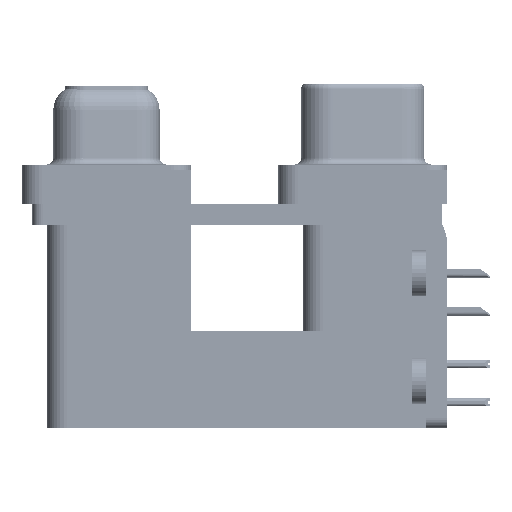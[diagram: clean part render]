
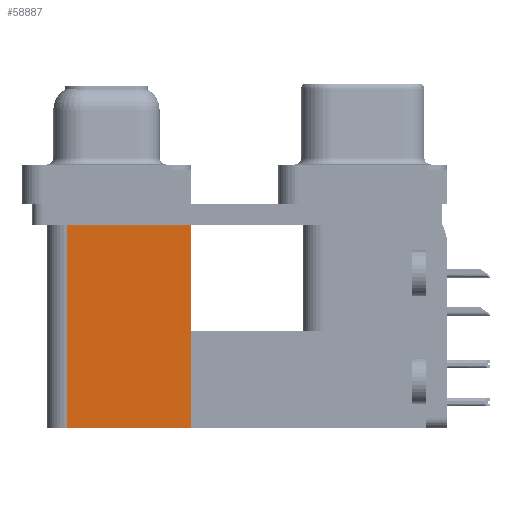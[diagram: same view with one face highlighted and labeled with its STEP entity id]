
A CAD part, left-side view. The second image highlights one B-rep face of the part: STEP entity #58887.
In plain terms, the highlighted planar face has unit normal (-1, 0, 0).
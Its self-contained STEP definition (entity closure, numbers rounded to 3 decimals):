
#113 = CARTESIAN_POINT ( 'NONE',  ( 3.79, 12.775, -19.2 ) ) ;
#594 = VECTOR ( 'NONE', #69800, 1000. ) ;
#6363 = VERTEX_POINT ( 'NONE', #7071 ) ;
#7071 = CARTESIAN_POINT ( 'NONE',  ( 3.79, 21.975, -2.5 ) ) ;
#8855 = DIRECTION ( 'NONE',  ( 0., 1., 0. ) ) ;
#9341 = ORIENTED_EDGE ( 'NONE', *, *, #26535, .T. ) ;
#10146 = EDGE_CURVE ( 'NONE', #29169, #64016, #26181, .T. ) ;
#14301 = VECTOR ( 'NONE', #15058, 1000. ) ;
#15058 = DIRECTION ( 'NONE',  ( 0., 1., 0. ) ) ;
#17545 = EDGE_CURVE ( 'NONE', #29169, #58087, #57967, .T. ) ;
#20665 = VECTOR ( 'NONE', #47305, 1000. ) ;
#25655 = LINE ( 'NONE', #69628, #20665 ) ;
#26181 = LINE ( 'NONE', #37513, #594 ) ;
#26535 = EDGE_CURVE ( 'NONE', #64016, #6363, #37748, .T. ) ;
#28440 = ORIENTED_EDGE ( 'NONE', *, *, #54474, .F. ) ;
#29169 = VERTEX_POINT ( 'NONE', #113 ) ;
#31036 = CARTESIAN_POINT ( 'NONE',  ( 3.79, 21.975, -19.2 ) ) ;
#31324 = CARTESIAN_POINT ( 'NONE',  ( 3.79, 12.775, -19.2 ) ) ;
#31369 = CARTESIAN_POINT ( 'NONE',  ( 3.79, 12.775, -2.5 ) ) ;
#32266 = EDGE_LOOP ( 'NONE', ( #9341, #28440, #35335, #55738 ) ) ;
#35335 = ORIENTED_EDGE ( 'NONE', *, *, #17545, .F. ) ;
#35794 = FACE_OUTER_BOUND ( 'NONE', #32266, .T. ) ;
#36137 = CARTESIAN_POINT ( 'NONE',  ( 3.79, 12.775, -19.2 ) ) ;
#37513 = CARTESIAN_POINT ( 'NONE',  ( 3.79, 12.775, -19.2 ) ) ;
#37748 = LINE ( 'NONE', #31369, #14301 ) ;
#38933 = AXIS2_PLACEMENT_3D ( 'NONE', #36137, #58477, #8855 ) ;
#46799 = PLANE ( 'NONE',  #38933 ) ;
#47305 = DIRECTION ( 'NONE',  ( 0., 0., 1. ) ) ;
#49839 = VECTOR ( 'NONE', #57616, 1000. ) ;
#54474 = EDGE_CURVE ( 'NONE', #58087, #6363, #25655, .T. ) ;
#55738 = ORIENTED_EDGE ( 'NONE', *, *, #10146, .T. ) ;
#57616 = DIRECTION ( 'NONE',  ( 0., 1., 0. ) ) ;
#57967 = LINE ( 'NONE', #31324, #49839 ) ;
#58087 = VERTEX_POINT ( 'NONE', #31036 ) ;
#58477 = DIRECTION ( 'NONE',  ( 1., 0., 0. ) ) ;
#58887 = ADVANCED_FACE ( 'NONE', ( #35794 ), #46799, .F. ) ;
#62816 = CARTESIAN_POINT ( 'NONE',  ( 3.79, 12.775, -2.5 ) ) ;
#64016 = VERTEX_POINT ( 'NONE', #62816 ) ;
#69628 = CARTESIAN_POINT ( 'NONE',  ( 3.79, 21.975, -19.2 ) ) ;
#69800 = DIRECTION ( 'NONE',  ( 0., 0., 1. ) ) ;
